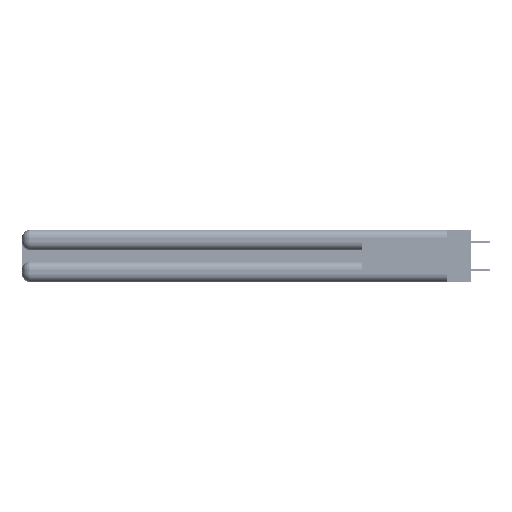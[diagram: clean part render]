
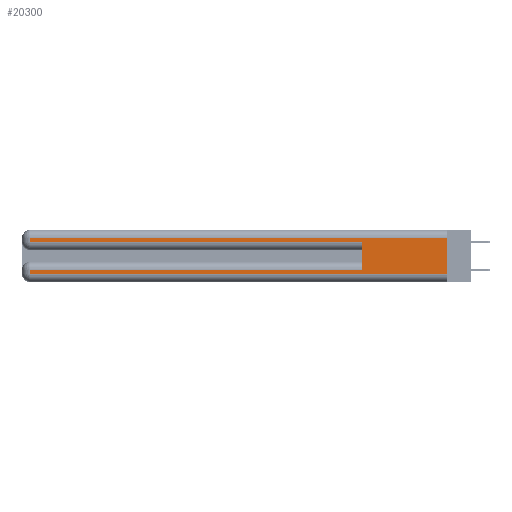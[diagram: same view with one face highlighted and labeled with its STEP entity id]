
A CAD part, left-side view. The second image highlights one B-rep face of the part: STEP entity #20300.
In plain terms, the highlighted planar face has unit normal (-1, 0, 0).
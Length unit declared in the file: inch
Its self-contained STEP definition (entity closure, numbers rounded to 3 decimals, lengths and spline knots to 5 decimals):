
#720 = CARTESIAN_POINT ( 'NONE',  ( 0., 0., 0.31 ) ) ;
#845 = CARTESIAN_POINT ( 'NONE',  ( 0., 2.94, 0.06 ) ) ;
#3068 = VECTOR ( 'NONE', #6115, 39.37008 ) ;
#3711 = ORIENTED_EDGE ( 'NONE', *, *, #49532, .T. ) ;
#3815 = CARTESIAN_POINT ( 'NONE',  ( 0., 0.6, 0.145 ) ) ;
#4151 = ORIENTED_EDGE ( 'NONE', *, *, #24477, .T. ) ;
#4440 = VERTEX_POINT ( 'NONE', #43565 ) ;
#4521 = EDGE_CURVE ( 'NONE', #14186, #38807, #52459, .T. ) ;
#5910 = DIRECTION ( 'NONE',  ( 0., 0., -1. ) ) ;
#6115 = DIRECTION ( 'NONE',  ( 0., 0., -1. ) ) ;
#6264 = EDGE_CURVE ( 'NONE', #21375, #11684, #26903, .T. ) ;
#7337 = ORIENTED_EDGE ( 'NONE', *, *, #45607, .T. ) ;
#7854 = CARTESIAN_POINT ( 'NONE',  ( 0., 0.6, 0.285 ) ) ;
#7858 = CARTESIAN_POINT ( 'NONE',  ( 0., 0., 0.06 ) ) ;
#7889 = VECTOR ( 'NONE', #36262, 39.37008 ) ;
#10052 = DIRECTION ( 'NONE',  ( 0., -1., 0. ) ) ;
#11050 = ORIENTED_EDGE ( 'NONE', *, *, #30381, .T. ) ;
#11070 = LINE ( 'NONE', #27810, #41775 ) ;
#11351 = DIRECTION ( 'NONE',  ( 0., 1., 0. ) ) ;
#11684 = VERTEX_POINT ( 'NONE', #845 ) ;
#12081 = LINE ( 'NONE', #32338, #25341 ) ;
#13735 = VECTOR ( 'NONE', #5910, 39.37008 ) ;
#14186 = VERTEX_POINT ( 'NONE', #720 ) ;
#14576 = DIRECTION ( 'NONE',  ( 1., 0., 0. ) ) ;
#15687 = AXIS2_PLACEMENT_3D ( 'NONE', #23462, #14576, #40234 ) ;
#19334 = VECTOR ( 'NONE', #20270, 39.37008 ) ;
#19779 = CARTESIAN_POINT ( 'NONE',  ( 0., 0., 0.37 ) ) ;
#20270 = DIRECTION ( 'NONE',  ( 0., 0., 1. ) ) ;
#20300 = ADVANCED_FACE ( 'NONE', ( #27777 ), #35125, .F. ) ;
#21375 = VERTEX_POINT ( 'NONE', #39307 ) ;
#22185 = ORIENTED_EDGE ( 'NONE', *, *, #49607, .F. ) ;
#22296 = ORIENTED_EDGE ( 'NONE', *, *, #6264, .T. ) ;
#23021 = CARTESIAN_POINT ( 'NONE',  ( 0., 0., 0.285 ) ) ;
#23106 = CARTESIAN_POINT ( 'NONE',  ( 0., 2.94, 0.37 ) ) ;
#23462 = CARTESIAN_POINT ( 'NONE',  ( 0., 0., 0.37 ) ) ;
#24477 = EDGE_CURVE ( 'NONE', #51670, #21375, #12081, .T. ) ;
#25341 = VECTOR ( 'NONE', #41552, 39.37008 ) ;
#25495 = LINE ( 'NONE', #42283, #36274 ) ;
#26426 = LINE ( 'NONE', #42944, #13735 ) ;
#26614 = CARTESIAN_POINT ( 'NONE',  ( 0., 2.94, 0.31 ) ) ;
#26903 = LINE ( 'NONE', #23106, #3068 ) ;
#27777 = FACE_OUTER_BOUND ( 'NONE', #38638, .T. ) ;
#27810 = CARTESIAN_POINT ( 'NONE',  ( 0., 0., 0.31 ) ) ;
#28087 = LINE ( 'NONE', #3815, #19334 ) ;
#28296 = CARTESIAN_POINT ( 'NONE',  ( 0., 0.6, 0.085 ) ) ;
#28331 = ORIENTED_EDGE ( 'NONE', *, *, #4521, .F. ) ;
#29006 = VERTEX_POINT ( 'NONE', #7854 ) ;
#29828 = DIRECTION ( 'NONE',  ( 0., -1., 0. ) ) ;
#30381 = EDGE_CURVE ( 'NONE', #4440, #29006, #43594, .T. ) ;
#32338 = CARTESIAN_POINT ( 'NONE',  ( 0., 0., 0.085 ) ) ;
#32641 = EDGE_CURVE ( 'NONE', #45417, #4440, #26426, .T. ) ;
#35125 = PLANE ( 'NONE',  #15687 ) ;
#36262 = DIRECTION ( 'NONE',  ( 0., 0., -1. ) ) ;
#36274 = VECTOR ( 'NONE', #29828, 39.37008 ) ;
#38638 = EDGE_LOOP ( 'NONE', ( #28331, #3711, #41682, #11050, #22185, #4151, #22296, #7337 ) ) ;
#38807 = VERTEX_POINT ( 'NONE', #7858 ) ;
#39307 = CARTESIAN_POINT ( 'NONE',  ( 0., 2.94, 0.085 ) ) ;
#39490 = VECTOR ( 'NONE', #10052, 39.37008 ) ;
#40234 = DIRECTION ( 'NONE',  ( 0., 0., -1. ) ) ;
#41552 = DIRECTION ( 'NONE',  ( 0., 1., 0. ) ) ;
#41682 = ORIENTED_EDGE ( 'NONE', *, *, #32641, .T. ) ;
#41775 = VECTOR ( 'NONE', #11351, 39.37008 ) ;
#42283 = CARTESIAN_POINT ( 'NONE',  ( 0., 0., 0.06 ) ) ;
#42944 = CARTESIAN_POINT ( 'NONE',  ( 0., 2.94, 0.37 ) ) ;
#43565 = CARTESIAN_POINT ( 'NONE',  ( 0., 2.94, 0.285 ) ) ;
#43594 = LINE ( 'NONE', #23021, #39490 ) ;
#45417 = VERTEX_POINT ( 'NONE', #26614 ) ;
#45607 = EDGE_CURVE ( 'NONE', #11684, #38807, #25495, .T. ) ;
#49532 = EDGE_CURVE ( 'NONE', #14186, #45417, #11070, .T. ) ;
#49607 = EDGE_CURVE ( 'NONE', #51670, #29006, #28087, .T. ) ;
#51670 = VERTEX_POINT ( 'NONE', #28296 ) ;
#52459 = LINE ( 'NONE', #19779, #7889 ) ;
